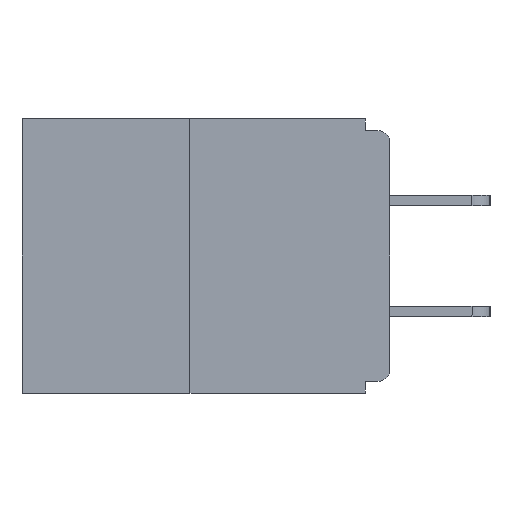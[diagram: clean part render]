
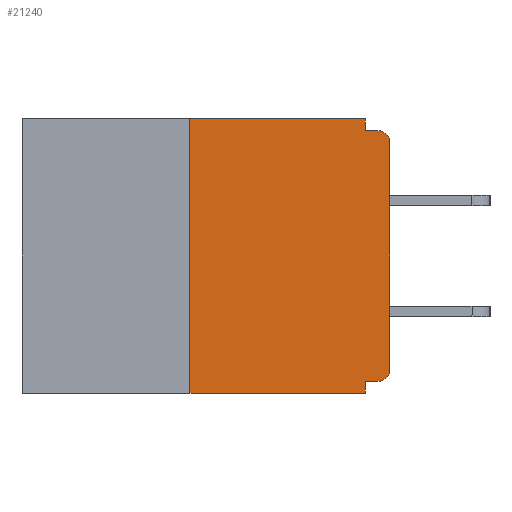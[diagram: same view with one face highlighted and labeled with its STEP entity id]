
A CAD part, left-side view. The second image highlights one B-rep face of the part: STEP entity #21240.
In plain terms, the highlighted planar face has unit normal (-1, 0, 0).
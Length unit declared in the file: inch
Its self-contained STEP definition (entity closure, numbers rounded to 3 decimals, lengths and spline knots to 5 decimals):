
#241 = EDGE_CURVE ( 'NONE', #24121, #16141, #22490, .T. ) ;
#891 = CARTESIAN_POINT ( 'NONE',  ( 0., 0., -0.328 ) ) ;
#957 = CARTESIAN_POINT ( 'NONE',  ( 0., 0.031, -0.343 ) ) ;
#1251 = CARTESIAN_POINT ( 'NONE',  ( 0., 0.25, 0. ) ) ;
#1394 = ORIENTED_EDGE ( 'NONE', *, *, #22353, .F. ) ;
#1466 = CARTESIAN_POINT ( 'NONE',  ( 0., 0.015, -0.328 ) ) ;
#1519 = DIRECTION ( 'NONE',  ( 0., 0., -1. ) ) ;
#1583 = CARTESIAN_POINT ( 'NONE',  ( 0., 0.015, -0.03 ) ) ;
#1636 = DIRECTION ( 'NONE',  ( 0., 0., -1. ) ) ;
#1865 = EDGE_LOOP ( 'NONE', ( #21576, #1394, #5645, #26519, #11150, #2573, #25775, #19189, #25437, #15176 ) ) ;
#1934 = DIRECTION ( 'NONE',  ( 0., -1., 0. ) ) ;
#2573 = ORIENTED_EDGE ( 'NONE', *, *, #16558, .T. ) ;
#2739 = EDGE_CURVE ( 'NONE', #17158, #16141, #10787, .T. ) ;
#3617 = AXIS2_PLACEMENT_3D ( 'NONE', #17201, #3744, #1636 ) ;
#3725 = CARTESIAN_POINT ( 'NONE',  ( 0., 0.031, 0. ) ) ;
#3744 = DIRECTION ( 'NONE',  ( -1., 0., 0. ) ) ;
#4079 = LINE ( 'NONE', #5161, #10566 ) ;
#4225 = VERTEX_POINT ( 'NONE', #1466 ) ;
#5161 = CARTESIAN_POINT ( 'NONE',  ( 0., 0.031, -0.343 ) ) ;
#5473 = DIRECTION ( 'NONE',  ( 0., 0., 1. ) ) ;
#5645 = ORIENTED_EDGE ( 'NONE', *, *, #19052, .T. ) ;
#6121 = VECTOR ( 'NONE', #11983, 39.37008 ) ;
#6374 = VECTOR ( 'NONE', #16121, 39.37008 ) ;
#6450 = EDGE_CURVE ( 'NONE', #10083, #17158, #18661, .T. ) ;
#6579 = FACE_OUTER_BOUND ( 'NONE', #1865, .T. ) ;
#6775 = CARTESIAN_POINT ( 'NONE',  ( 0., 0.031, -0.328 ) ) ;
#7321 = CARTESIAN_POINT ( 'NONE',  ( 0., 0., -0.03 ) ) ;
#7919 = LINE ( 'NONE', #16338, #13355 ) ;
#8600 = CARTESIAN_POINT ( 'NONE',  ( 0., 0.031, -0.015 ) ) ;
#9222 = CARTESIAN_POINT ( 'NONE',  ( 0., 0.015, -0.015 ) ) ;
#9415 = LINE ( 'NONE', #3725, #22362 ) ;
#10083 = VERTEX_POINT ( 'NONE', #13679 ) ;
#10566 = VECTOR ( 'NONE', #20428, 39.37008 ) ;
#10787 = CIRCLE ( 'NONE', #18251, 0.015 ) ;
#10827 = CARTESIAN_POINT ( 'NONE',  ( 0., 0.25, -0.343 ) ) ;
#10926 = EDGE_CURVE ( 'NONE', #25620, #24121, #9415, .T. ) ;
#11150 = ORIENTED_EDGE ( 'NONE', *, *, #14596, .F. ) ;
#11983 = DIRECTION ( 'NONE',  ( 0., 1., 0. ) ) ;
#12776 = VERTEX_POINT ( 'NONE', #1251 ) ;
#13355 = VECTOR ( 'NONE', #5473, 39.37008 ) ;
#13679 = CARTESIAN_POINT ( 'NONE',  ( 0., 0., -0.313 ) ) ;
#14248 = EDGE_CURVE ( 'NONE', #20890, #14847, #4079, .T. ) ;
#14328 = VECTOR ( 'NONE', #18869, 39.37008 ) ;
#14596 = EDGE_CURVE ( 'NONE', #4225, #20890, #24856, .T. ) ;
#14847 = VERTEX_POINT ( 'NONE', #957 ) ;
#15176 = ORIENTED_EDGE ( 'NONE', *, *, #10926, .F. ) ;
#15222 = VECTOR ( 'NONE', #24335, 39.37008 ) ;
#15306 = VERTEX_POINT ( 'NONE', #10827 ) ;
#15511 = CARTESIAN_POINT ( 'NONE',  ( 0., 0.031, 0. ) ) ;
#16062 = LINE ( 'NONE', #24108, #27318 ) ;
#16121 = DIRECTION ( 'NONE',  ( 0., 0., 1. ) ) ;
#16141 = VERTEX_POINT ( 'NONE', #9222 ) ;
#16338 = CARTESIAN_POINT ( 'NONE',  ( 0., 0.25, 0. ) ) ;
#16558 = EDGE_CURVE ( 'NONE', #4225, #10083, #19798, .T. ) ;
#16837 = CARTESIAN_POINT ( 'NONE',  ( 0., 0.46, 0. ) ) ;
#16842 = AXIS2_PLACEMENT_3D ( 'NONE', #16837, #23388, #19049 ) ;
#17158 = VERTEX_POINT ( 'NONE', #7321 ) ;
#17201 = CARTESIAN_POINT ( 'NONE',  ( 0., 0.015, -0.313 ) ) ;
#18195 = CARTESIAN_POINT ( 'NONE',  ( 0., 0., -0.015 ) ) ;
#18251 = AXIS2_PLACEMENT_3D ( 'NONE', #1583, #20887, #21245 ) ;
#18661 = LINE ( 'NONE', #26980, #6374 ) ;
#18869 = DIRECTION ( 'NONE',  ( 0., -1., 0. ) ) ;
#19049 = DIRECTION ( 'NONE',  ( 0., 0., -1. ) ) ;
#19052 = EDGE_CURVE ( 'NONE', #15306, #14847, #21047, .T. ) ;
#19189 = ORIENTED_EDGE ( 'NONE', *, *, #2739, .T. ) ;
#19798 = CIRCLE ( 'NONE', #3617, 0.015 ) ;
#20428 = DIRECTION ( 'NONE',  ( 0., 0., -1. ) ) ;
#20887 = DIRECTION ( 'NONE',  ( -1., 0., 0. ) ) ;
#20890 = VERTEX_POINT ( 'NONE', #6775 ) ;
#21047 = LINE ( 'NONE', #26620, #15222 ) ;
#21240 = ADVANCED_FACE ( 'NONE', ( #6579 ), #25593, .F. ) ;
#21245 = DIRECTION ( 'NONE',  ( 0., 0., -1. ) ) ;
#21576 = ORIENTED_EDGE ( 'NONE', *, *, #22649, .F. ) ;
#22353 = EDGE_CURVE ( 'NONE', #15306, #12776, #7919, .T. ) ;
#22362 = VECTOR ( 'NONE', #1519, 39.37008 ) ;
#22490 = LINE ( 'NONE', #18195, #14328 ) ;
#22649 = EDGE_CURVE ( 'NONE', #12776, #25620, #16062, .T. ) ;
#23388 = DIRECTION ( 'NONE',  ( 1., 0., 0. ) ) ;
#24108 = CARTESIAN_POINT ( 'NONE',  ( 0., 0.46, 0. ) ) ;
#24121 = VERTEX_POINT ( 'NONE', #8600 ) ;
#24335 = DIRECTION ( 'NONE',  ( 0., -1., 0. ) ) ;
#24856 = LINE ( 'NONE', #891, #6121 ) ;
#25437 = ORIENTED_EDGE ( 'NONE', *, *, #241, .F. ) ;
#25593 = PLANE ( 'NONE',  #16842 ) ;
#25620 = VERTEX_POINT ( 'NONE', #15511 ) ;
#25775 = ORIENTED_EDGE ( 'NONE', *, *, #6450, .T. ) ;
#26519 = ORIENTED_EDGE ( 'NONE', *, *, #14248, .F. ) ;
#26620 = CARTESIAN_POINT ( 'NONE',  ( 0., 0.46, -0.343 ) ) ;
#26980 = CARTESIAN_POINT ( 'NONE',  ( 0., 0., 0. ) ) ;
#27318 = VECTOR ( 'NONE', #1934, 39.37008 ) ;
